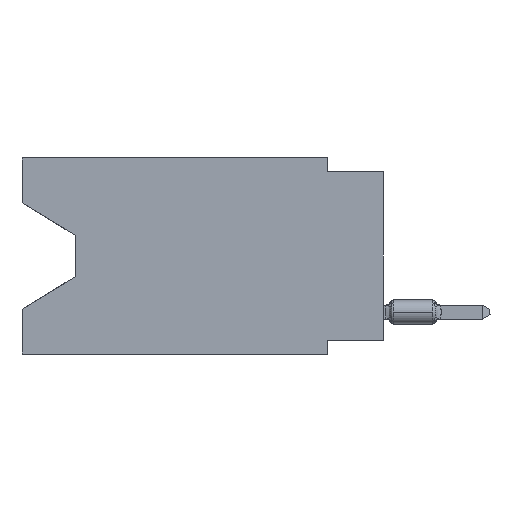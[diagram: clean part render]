
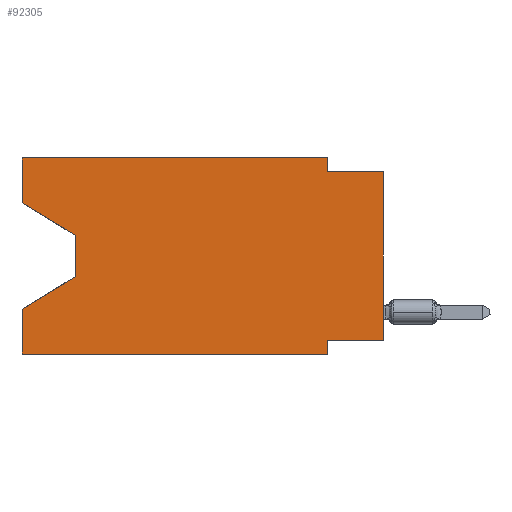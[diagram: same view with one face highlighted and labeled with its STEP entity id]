
A CAD part, left-side view. The second image highlights one B-rep face of the part: STEP entity #92305.
In plain terms, the highlighted planar face has unit normal (-1, 0, 0).
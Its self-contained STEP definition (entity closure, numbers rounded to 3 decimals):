
#51 = LINE ( 'NONE', #8175, #14693 ) ;
#399 = LINE ( 'NONE', #24793, #54065 ) ;
#2195 = ORIENTED_EDGE ( 'NONE', *, *, #10731, .F. ) ;
#2557 = VECTOR ( 'NONE', #35621, 1000. ) ;
#2771 = VERTEX_POINT ( 'NONE', #67293 ) ;
#2873 = ORIENTED_EDGE ( 'NONE', *, *, #47413, .T. ) ;
#5487 = LINE ( 'NONE', #15195, #30236 ) ;
#5748 = CARTESIAN_POINT ( 'NONE',  ( 0., 13.97, -3.505 ) ) ;
#6009 = DIRECTION ( 'NONE',  ( 0., 0., 1. ) ) ;
#6037 = CARTESIAN_POINT ( 'NONE',  ( 0., 16.383, 0. ) ) ;
#7118 = CARTESIAN_POINT ( 'NONE',  ( 0., 13.97, -5.385 ) ) ;
#8175 = CARTESIAN_POINT ( 'NONE',  ( 0., 16.383, -8.89 ) ) ;
#8587 = VECTOR ( 'NONE', #93838, 1000. ) ;
#10022 = CARTESIAN_POINT ( 'NONE',  ( 0., 16.383, -2.038 ) ) ;
#10731 = EDGE_CURVE ( 'NONE', #19532, #16786, #60754, .T. ) ;
#11178 = LINE ( 'NONE', #68706, #2557 ) ;
#13707 = VERTEX_POINT ( 'NONE', #107173 ) ;
#14693 = VECTOR ( 'NONE', #49929, 1000. ) ;
#14918 = LINE ( 'NONE', #5748, #97929 ) ;
#14989 = ORIENTED_EDGE ( 'NONE', *, *, #35442, .F. ) ;
#15195 = CARTESIAN_POINT ( 'NONE',  ( 0., 0., 0. ) ) ;
#15406 = CARTESIAN_POINT ( 'NONE',  ( 0., 2.54, -0.635 ) ) ;
#16786 = VERTEX_POINT ( 'NONE', #93059 ) ;
#18412 = CARTESIAN_POINT ( 'NONE',  ( 0., 13.97, -5.385 ) ) ;
#19532 = VERTEX_POINT ( 'NONE', #15406 ) ;
#22828 = VECTOR ( 'NONE', #42984, 1000. ) ;
#24461 = LINE ( 'NONE', #50477, #48159 ) ;
#24793 = CARTESIAN_POINT ( 'NONE',  ( 0., 16.383, 0. ) ) ;
#27053 = ORIENTED_EDGE ( 'NONE', *, *, #54010, .T. ) ;
#27651 = CARTESIAN_POINT ( 'NONE',  ( 0., 0., -0.635 ) ) ;
#28765 = ORIENTED_EDGE ( 'NONE', *, *, #48678, .F. ) ;
#29897 = CARTESIAN_POINT ( 'NONE',  ( 0., 16.383, 0. ) ) ;
#30236 = VECTOR ( 'NONE', #6009, 1000. ) ;
#30787 = ORIENTED_EDGE ( 'NONE', *, *, #100669, .F. ) ;
#32592 = PLANE ( 'NONE',  #95952 ) ;
#33032 = EDGE_CURVE ( 'NONE', #2771, #16786, #5487, .T. ) ;
#33168 = CARTESIAN_POINT ( 'NONE',  ( 0., 16.383, -6.852 ) ) ;
#34703 = DIRECTION ( 'NONE',  ( 0., 0.855, -0.519 ) ) ;
#35216 = LINE ( 'NONE', #68302, #68194 ) ;
#35442 = EDGE_CURVE ( 'NONE', #93861, #96019, #70621, .T. ) ;
#35621 = DIRECTION ( 'NONE',  ( 0., -0.855, -0.519 ) ) ;
#38590 = DIRECTION ( 'NONE',  ( 1., 0., 0. ) ) ;
#39219 = EDGE_CURVE ( 'NONE', #72153, #13707, #51, .T. ) ;
#40760 = CARTESIAN_POINT ( 'NONE',  ( 0., 2.54, -8.255 ) ) ;
#41148 = EDGE_CURVE ( 'NONE', #81864, #44486, #14918, .T. ) ;
#42984 = DIRECTION ( 'NONE',  ( 0., 0., -1. ) ) ;
#43897 = EDGE_LOOP ( 'NONE', ( #27053, #106416, #2873, #60549, #60822, #56398, #76155, #100961, #2195, #30787, #14989, #28765 ) ) ;
#44486 = VERTEX_POINT ( 'NONE', #7118 ) ;
#47413 = EDGE_CURVE ( 'NONE', #44486, #80451, #58604, .T. ) ;
#48159 = VECTOR ( 'NONE', #75441, 1000. ) ;
#48284 = EDGE_CURVE ( 'NONE', #70294, #13707, #75556, .T. ) ;
#48678 = EDGE_CURVE ( 'NONE', #82020, #93861, #399, .T. ) ;
#49929 = DIRECTION ( 'NONE',  ( 0., -1., 0. ) ) ;
#49955 = VECTOR ( 'NONE', #88492, 1000. ) ;
#50477 = CARTESIAN_POINT ( 'NONE',  ( 0., 16.383, 0. ) ) ;
#52970 = LINE ( 'NONE', #71408, #73611 ) ;
#54010 = EDGE_CURVE ( 'NONE', #82020, #81864, #11178, .T. ) ;
#54065 = VECTOR ( 'NONE', #91512, 1000. ) ;
#56398 = ORIENTED_EDGE ( 'NONE', *, *, #48284, .F. ) ;
#58604 = LINE ( 'NONE', #18412, #67792 ) ;
#60549 = ORIENTED_EDGE ( 'NONE', *, *, #83872, .F. ) ;
#60754 = LINE ( 'NONE', #27651, #8587 ) ;
#60822 = ORIENTED_EDGE ( 'NONE', *, *, #39219, .T. ) ;
#61649 = DIRECTION ( 'NONE',  ( 0., 1., 0. ) ) ;
#64425 = CARTESIAN_POINT ( 'NONE',  ( 0., 16.383, -8.89 ) ) ;
#65677 = DIRECTION ( 'NONE',  ( 0., 0., -1. ) ) ;
#67293 = CARTESIAN_POINT ( 'NONE',  ( 0., 0., -8.255 ) ) ;
#67792 = VECTOR ( 'NONE', #34703, 1000. ) ;
#68194 = VECTOR ( 'NONE', #101365, 1000. ) ;
#68302 = CARTESIAN_POINT ( 'NONE',  ( 0., 2.54, 0. ) ) ;
#68706 = CARTESIAN_POINT ( 'NONE',  ( 0., 16.383, -2.038 ) ) ;
#70294 = VERTEX_POINT ( 'NONE', #40760 ) ;
#70621 = LINE ( 'NONE', #87969, #49955 ) ;
#71408 = CARTESIAN_POINT ( 'NONE',  ( 0., 0., -8.255 ) ) ;
#72153 = VERTEX_POINT ( 'NONE', #64425 ) ;
#73564 = CARTESIAN_POINT ( 'NONE',  ( 0., 2.54, 0. ) ) ;
#73611 = VECTOR ( 'NONE', #61649, 1000. ) ;
#74782 = CARTESIAN_POINT ( 'NONE',  ( 0., 13.97, -3.505 ) ) ;
#75441 = DIRECTION ( 'NONE',  ( 0., 0., 1. ) ) ;
#75556 = LINE ( 'NONE', #76624, #22828 ) ;
#76155 = ORIENTED_EDGE ( 'NONE', *, *, #91396, .F. ) ;
#76624 = CARTESIAN_POINT ( 'NONE',  ( 0., 2.54, -8.89 ) ) ;
#80451 = VERTEX_POINT ( 'NONE', #33168 ) ;
#81864 = VERTEX_POINT ( 'NONE', #74782 ) ;
#82020 = VERTEX_POINT ( 'NONE', #10022 ) ;
#83872 = EDGE_CURVE ( 'NONE', #72153, #80451, #24461, .T. ) ;
#87954 = FACE_OUTER_BOUND ( 'NONE', #43897, .T. ) ;
#87969 = CARTESIAN_POINT ( 'NONE',  ( 0., 16.383, 0. ) ) ;
#88492 = DIRECTION ( 'NONE',  ( 0., -1., 0. ) ) ;
#89789 = DIRECTION ( 'NONE',  ( 0., 0., -1. ) ) ;
#91396 = EDGE_CURVE ( 'NONE', #2771, #70294, #52970, .T. ) ;
#91512 = DIRECTION ( 'NONE',  ( 0., 0., 1. ) ) ;
#92305 = ADVANCED_FACE ( 'NONE', ( #87954 ), #32592, .F. ) ;
#93059 = CARTESIAN_POINT ( 'NONE',  ( 0., 0., -0.635 ) ) ;
#93838 = DIRECTION ( 'NONE',  ( 0., -1., 0. ) ) ;
#93861 = VERTEX_POINT ( 'NONE', #29897 ) ;
#95952 = AXIS2_PLACEMENT_3D ( 'NONE', #6037, #38590, #65677 ) ;
#96019 = VERTEX_POINT ( 'NONE', #73564 ) ;
#97929 = VECTOR ( 'NONE', #89789, 1000. ) ;
#100669 = EDGE_CURVE ( 'NONE', #96019, #19532, #35216, .T. ) ;
#100961 = ORIENTED_EDGE ( 'NONE', *, *, #33032, .T. ) ;
#101365 = DIRECTION ( 'NONE',  ( 0., 0., -1. ) ) ;
#106416 = ORIENTED_EDGE ( 'NONE', *, *, #41148, .T. ) ;
#107173 = CARTESIAN_POINT ( 'NONE',  ( 0., 2.54, -8.89 ) ) ;
